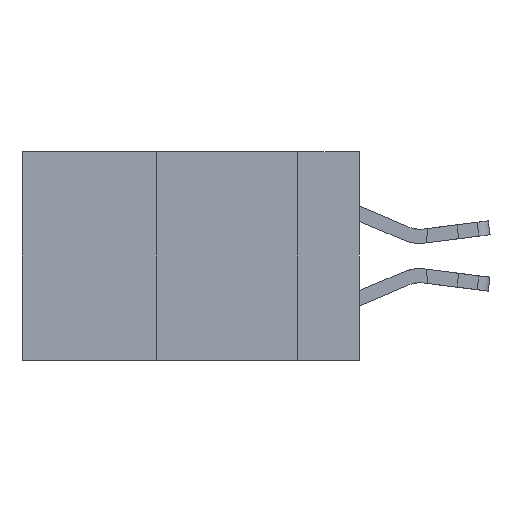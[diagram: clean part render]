
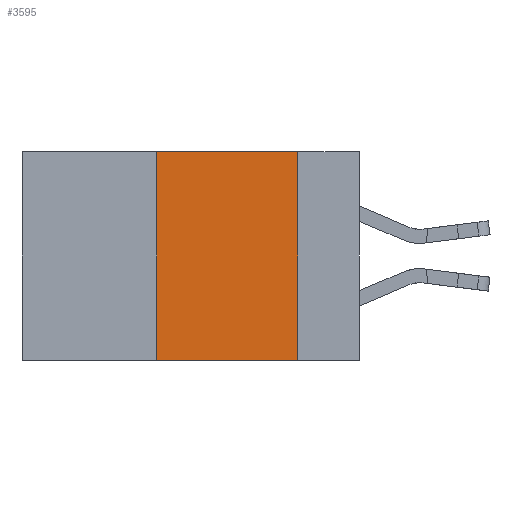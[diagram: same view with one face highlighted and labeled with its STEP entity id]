
A CAD part, left-side view. The second image highlights one B-rep face of the part: STEP entity #3595.
In plain terms, the highlighted planar face has unit normal (-1, 0, 0).
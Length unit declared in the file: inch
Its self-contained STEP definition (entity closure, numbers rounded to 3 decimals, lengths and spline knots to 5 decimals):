
#807 = DIRECTION ( 'NONE',  ( 0., -1., 0. ) ) ;
#821 = ORIENTED_EDGE ( 'NONE', *, *, #15518, .F. ) ;
#1805 = EDGE_LOOP ( 'NONE', ( #7254, #821, #13895, #12188 ) ) ;
#2137 = CARTESIAN_POINT ( 'NONE',  ( 0., 0.6, 0. ) ) ;
#2611 = DIRECTION ( 'NONE',  ( 0., 0., 1. ) ) ;
#2653 = LINE ( 'NONE', #12027, #16580 ) ;
#3185 = EDGE_CURVE ( 'NONE', #16424, #6247, #9017, .T. ) ;
#3595 = ADVANCED_FACE ( 'NONE', ( #13340 ), #17174, .F. ) ;
#3957 = CARTESIAN_POINT ( 'NONE',  ( 0., 0.36, 0. ) ) ;
#4939 = CARTESIAN_POINT ( 'NONE',  ( 0., 0.11, -0.37 ) ) ;
#6134 = CARTESIAN_POINT ( 'NONE',  ( 0., 0.6, 0. ) ) ;
#6217 = DIRECTION ( 'NONE',  ( 1., 0., 0. ) ) ;
#6247 = VERTEX_POINT ( 'NONE', #4939 ) ;
#6592 = EDGE_CURVE ( 'NONE', #14665, #6247, #2653, .T. ) ;
#7254 = ORIENTED_EDGE ( 'NONE', *, *, #6592, .F. ) ;
#7699 = CARTESIAN_POINT ( 'NONE',  ( 0., 0.11, 0. ) ) ;
#7951 = VECTOR ( 'NONE', #2611, 39.37008 ) ;
#9017 = LINE ( 'NONE', #14429, #10912 ) ;
#10707 = DIRECTION ( 'NONE',  ( 0., -1., 0. ) ) ;
#10756 = LINE ( 'NONE', #3957, #7951 ) ;
#10912 = VECTOR ( 'NONE', #10707, 39.37008 ) ;
#11544 = CARTESIAN_POINT ( 'NONE',  ( 0., 0.36, -0.37 ) ) ;
#11648 = VECTOR ( 'NONE', #807, 39.37008 ) ;
#11926 = DIRECTION ( 'NONE',  ( 0., 0., -1. ) ) ;
#12027 = CARTESIAN_POINT ( 'NONE',  ( 0., 0.11, 0. ) ) ;
#12188 = ORIENTED_EDGE ( 'NONE', *, *, #3185, .T. ) ;
#13340 = FACE_OUTER_BOUND ( 'NONE', #1805, .T. ) ;
#13895 = ORIENTED_EDGE ( 'NONE', *, *, #16166, .F. ) ;
#14429 = CARTESIAN_POINT ( 'NONE',  ( 0., 0.6, -0.37 ) ) ;
#14665 = VERTEX_POINT ( 'NONE', #7699 ) ;
#15148 = CARTESIAN_POINT ( 'NONE',  ( 0., 0.36, 0. ) ) ;
#15367 = VERTEX_POINT ( 'NONE', #15148 ) ;
#15518 = EDGE_CURVE ( 'NONE', #15367, #14665, #16928, .T. ) ;
#15915 = AXIS2_PLACEMENT_3D ( 'NONE', #6134, #6217, #11926 ) ;
#16166 = EDGE_CURVE ( 'NONE', #16424, #15367, #10756, .T. ) ;
#16424 = VERTEX_POINT ( 'NONE', #11544 ) ;
#16580 = VECTOR ( 'NONE', #17533, 39.37008 ) ;
#16928 = LINE ( 'NONE', #2137, #11648 ) ;
#17174 = PLANE ( 'NONE',  #15915 ) ;
#17533 = DIRECTION ( 'NONE',  ( 0., 0., -1. ) ) ;
